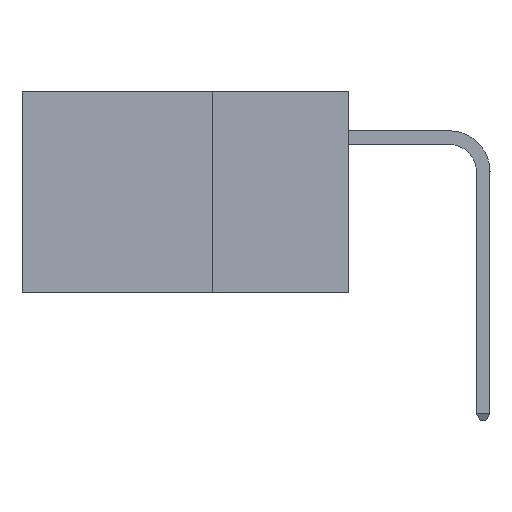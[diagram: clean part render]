
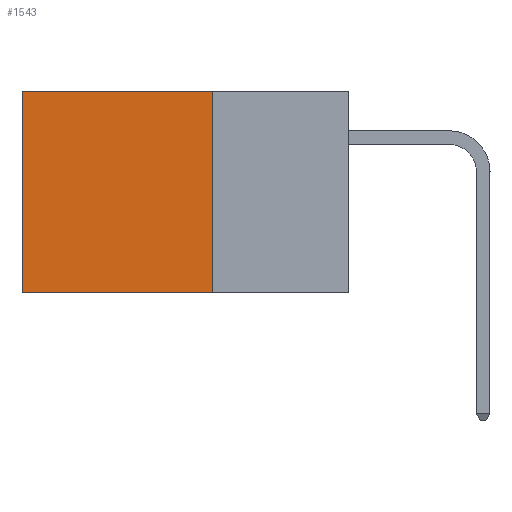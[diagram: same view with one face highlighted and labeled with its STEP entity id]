
A CAD part, left-side view. The second image highlights one B-rep face of the part: STEP entity #1543.
In plain terms, the highlighted planar face has unit normal (-1, 0, 0).
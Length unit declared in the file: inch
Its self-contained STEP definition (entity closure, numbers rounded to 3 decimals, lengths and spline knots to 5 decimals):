
#457 = CARTESIAN_POINT ( 'NONE',  ( 0.2875, 0.25, 0. ) ) ;
#564 = EDGE_CURVE ( 'NONE', #17121, #11106, #12931, .T. ) ;
#580 = EDGE_CURVE ( 'NONE', #17121, #13673, #6732, .T. ) ;
#649 = DIRECTION ( 'NONE',  ( 0., 0., -1. ) ) ;
#1543 = ADVANCED_FACE ( 'NONE', ( #18750 ), #9172, .F. ) ;
#2473 = CARTESIAN_POINT ( 'NONE',  ( 0.2875, 0.6, 0. ) ) ;
#2640 = EDGE_CURVE ( 'NONE', #13673, #9876, #4005, .T. ) ;
#2743 = CARTESIAN_POINT ( 'NONE',  ( 0.2875, 0.25, 0. ) ) ;
#2744 = VECTOR ( 'NONE', #649, 39.37008 ) ;
#2875 = DIRECTION ( 'NONE',  ( 0., 1., 0. ) ) ;
#3250 = CARTESIAN_POINT ( 'NONE',  ( 0.2875, 0.25, -0.37 ) ) ;
#3380 = ORIENTED_EDGE ( 'NONE', *, *, #19825, .F. ) ;
#4005 = LINE ( 'NONE', #2473, #18504 ) ;
#4426 = CARTESIAN_POINT ( 'NONE',  ( 0.2875, 0.25, -0.37 ) ) ;
#5093 = CARTESIAN_POINT ( 'NONE',  ( 0.2875, 0.25, 0. ) ) ;
#5135 = ORIENTED_EDGE ( 'NONE', *, *, #564, .F. ) ;
#6732 = LINE ( 'NONE', #5093, #16898 ) ;
#6923 = DIRECTION ( 'NONE',  ( 0., 1., 0. ) ) ;
#7426 = ORIENTED_EDGE ( 'NONE', *, *, #2640, .T. ) ;
#9172 = PLANE ( 'NONE',  #12692 ) ;
#9876 = VERTEX_POINT ( 'NONE', #20160 ) ;
#10584 = EDGE_LOOP ( 'NONE', ( #7426, #3380, #5135, #16125 ) ) ;
#10914 = CARTESIAN_POINT ( 'NONE',  ( 0.2875, 0.25, 0. ) ) ;
#11106 = VERTEX_POINT ( 'NONE', #3250 ) ;
#12692 = AXIS2_PLACEMENT_3D ( 'NONE', #10914, #13503, #17201 ) ;
#12931 = LINE ( 'NONE', #457, #2744 ) ;
#13503 = DIRECTION ( 'NONE',  ( 1., 0., 0. ) ) ;
#13673 = VERTEX_POINT ( 'NONE', #14978 ) ;
#14978 = CARTESIAN_POINT ( 'NONE',  ( 0.2875, 0.6, 0. ) ) ;
#15263 = DIRECTION ( 'NONE',  ( 0., 0., -1. ) ) ;
#15699 = VECTOR ( 'NONE', #2875, 39.37008 ) ;
#16125 = ORIENTED_EDGE ( 'NONE', *, *, #580, .T. ) ;
#16898 = VECTOR ( 'NONE', #6923, 39.37008 ) ;
#17121 = VERTEX_POINT ( 'NONE', #2743 ) ;
#17201 = DIRECTION ( 'NONE',  ( 0., 0., -1. ) ) ;
#18504 = VECTOR ( 'NONE', #15263, 39.37008 ) ;
#18544 = LINE ( 'NONE', #4426, #15699 ) ;
#18750 = FACE_OUTER_BOUND ( 'NONE', #10584, .T. ) ;
#19825 = EDGE_CURVE ( 'NONE', #11106, #9876, #18544, .T. ) ;
#20160 = CARTESIAN_POINT ( 'NONE',  ( 0.2875, 0.6, -0.37 ) ) ;
